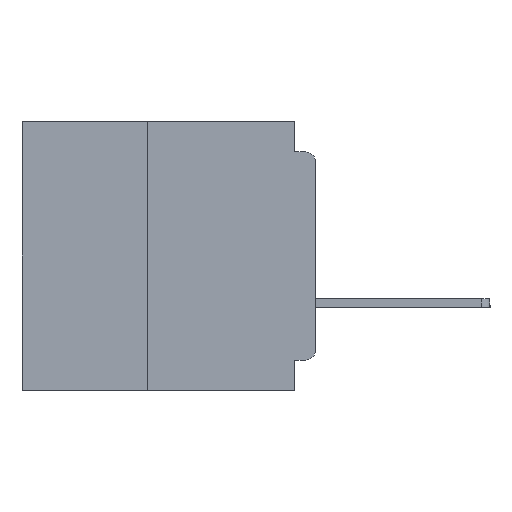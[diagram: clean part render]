
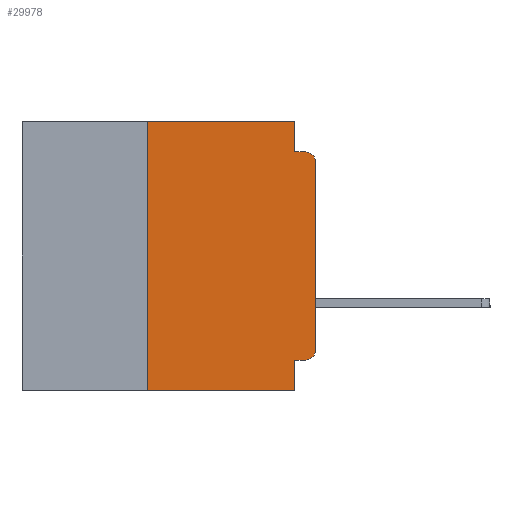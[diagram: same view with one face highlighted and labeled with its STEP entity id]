
A CAD part, left-side view. The second image highlights one B-rep face of the part: STEP entity #29978.
In plain terms, the highlighted planar face has unit normal (-1, 0, 0).
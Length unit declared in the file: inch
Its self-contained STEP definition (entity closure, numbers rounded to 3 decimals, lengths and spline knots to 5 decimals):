
#248 = VERTEX_POINT ( 'NONE', #37968 ) ;
#346 = LINE ( 'NONE', #29922, #40143 ) ;
#841 = CARTESIAN_POINT ( 'NONE',  ( 0., 0.015, -0.06 ) ) ;
#1533 = CARTESIAN_POINT ( 'NONE',  ( 0., 0.25, 0. ) ) ;
#1706 = ORIENTED_EDGE ( 'NONE', *, *, #34268, .T. ) ;
#2144 = EDGE_CURVE ( 'NONE', #54916, #248, #28563, .T. ) ;
#3180 = VECTOR ( 'NONE', #64614, 39.37008 ) ;
#4664 = ORIENTED_EDGE ( 'NONE', *, *, #55768, .F. ) ;
#5012 = CARTESIAN_POINT ( 'NONE',  ( 0., 0.015, -0.355 ) ) ;
#5513 = VECTOR ( 'NONE', #36241, 39.37008 ) ;
#5719 = VECTOR ( 'NONE', #46419, 39.37008 ) ;
#5851 = CARTESIAN_POINT ( 'NONE',  ( 0., 0.015, -0.045 ) ) ;
#6122 = DIRECTION ( 'NONE',  ( 0., 0., -1. ) ) ;
#8767 = LINE ( 'NONE', #56888, #5513 ) ;
#10810 = CARTESIAN_POINT ( 'NONE',  ( 0., 0., -0.06 ) ) ;
#13186 = VECTOR ( 'NONE', #66422, 39.37008 ) ;
#15886 = EDGE_CURVE ( 'NONE', #248, #17836, #17030, .T. ) ;
#16548 = DIRECTION ( 'NONE',  ( 1., 0., 0. ) ) ;
#17030 = LINE ( 'NONE', #44818, #20254 ) ;
#17603 = ORIENTED_EDGE ( 'NONE', *, *, #54045, .F. ) ;
#17836 = VERTEX_POINT ( 'NONE', #18059 ) ;
#18059 = CARTESIAN_POINT ( 'NONE',  ( 0., 0.031, -0.4 ) ) ;
#18312 = AXIS2_PLACEMENT_3D ( 'NONE', #22030, #58297, #27219 ) ;
#19252 = DIRECTION ( 'NONE',  ( 0., 0., -1. ) ) ;
#19547 = LINE ( 'NONE', #51428, #5719 ) ;
#20254 = VECTOR ( 'NONE', #19252, 39.37008 ) ;
#21035 = VERTEX_POINT ( 'NONE', #61242 ) ;
#22030 = CARTESIAN_POINT ( 'NONE',  ( 0., 0.015, -0.34 ) ) ;
#23277 = ORIENTED_EDGE ( 'NONE', *, *, #52004, .T. ) ;
#24165 = EDGE_CURVE ( 'NONE', #42145, #42224, #346, .T. ) ;
#26430 = VERTEX_POINT ( 'NONE', #1533 ) ;
#27219 = DIRECTION ( 'NONE',  ( 0., 0., -1. ) ) ;
#27846 = CARTESIAN_POINT ( 'NONE',  ( 0., 0.031, 0. ) ) ;
#28563 = LINE ( 'NONE', #45722, #13186 ) ;
#29922 = CARTESIAN_POINT ( 'NONE',  ( 0., 0., -0.045 ) ) ;
#29978 = ADVANCED_FACE ( 'NONE', ( #32818 ), #37120, .F. ) ;
#30312 = ORIENTED_EDGE ( 'NONE', *, *, #15886, .F. ) ;
#31312 = ORIENTED_EDGE ( 'NONE', *, *, #24165, .F. ) ;
#32818 = FACE_OUTER_BOUND ( 'NONE', #62826, .T. ) ;
#33409 = VECTOR ( 'NONE', #45079, 39.37008 ) ;
#34268 = EDGE_CURVE ( 'NONE', #21035, #17836, #8767, .T. ) ;
#34377 = VERTEX_POINT ( 'NONE', #10810 ) ;
#36174 = CIRCLE ( 'NONE', #65828, 0.015 ) ;
#36241 = DIRECTION ( 'NONE',  ( 0., -1., 0. ) ) ;
#36369 = EDGE_CURVE ( 'NONE', #21035, #26430, #41226, .T. ) ;
#37120 = PLANE ( 'NONE',  #41165 ) ;
#37164 = DIRECTION ( 'NONE',  ( -1., 0., 0. ) ) ;
#37672 = EDGE_CURVE ( 'NONE', #34377, #42224, #36174, .T. ) ;
#37968 = CARTESIAN_POINT ( 'NONE',  ( 0., 0.031, -0.355 ) ) ;
#39195 = ORIENTED_EDGE ( 'NONE', *, *, #55540, .T. ) ;
#40143 = VECTOR ( 'NONE', #55816, 39.37008 ) ;
#41165 = AXIS2_PLACEMENT_3D ( 'NONE', #47565, #16548, #52769 ) ;
#41226 = LINE ( 'NONE', #58347, #67251 ) ;
#42145 = VERTEX_POINT ( 'NONE', #46649 ) ;
#42224 = VERTEX_POINT ( 'NONE', #5851 ) ;
#44596 = LINE ( 'NONE', #58444, #3180 ) ;
#44760 = VERTEX_POINT ( 'NONE', #45017 ) ;
#44818 = CARTESIAN_POINT ( 'NONE',  ( 0., 0.031, -0.4 ) ) ;
#45017 = CARTESIAN_POINT ( 'NONE',  ( 0., 0., -0.34 ) ) ;
#45079 = DIRECTION ( 'NONE',  ( 0., -1., 0. ) ) ;
#45722 = CARTESIAN_POINT ( 'NONE',  ( 0., 0., -0.355 ) ) ;
#46419 = DIRECTION ( 'NONE',  ( 0., 0., 1. ) ) ;
#46649 = CARTESIAN_POINT ( 'NONE',  ( 0., 0.031, -0.045 ) ) ;
#47565 = CARTESIAN_POINT ( 'NONE',  ( 0., 0.437, 0. ) ) ;
#51428 = CARTESIAN_POINT ( 'NONE',  ( 0., 0., 0. ) ) ;
#52004 = EDGE_CURVE ( 'NONE', #54916, #44760, #58487, .T. ) ;
#52769 = DIRECTION ( 'NONE',  ( 0., 0., -1. ) ) ;
#54045 = EDGE_CURVE ( 'NONE', #26430, #66550, #64300, .T. ) ;
#54916 = VERTEX_POINT ( 'NONE', #5012 ) ;
#55540 = EDGE_CURVE ( 'NONE', #44760, #34377, #19547, .T. ) ;
#55768 = EDGE_CURVE ( 'NONE', #66550, #42145, #44596, .T. ) ;
#55816 = DIRECTION ( 'NONE',  ( 0., -1., 0. ) ) ;
#56888 = CARTESIAN_POINT ( 'NONE',  ( 0., 0.437, -0.4 ) ) ;
#58297 = DIRECTION ( 'NONE',  ( -1., 0., 0. ) ) ;
#58347 = CARTESIAN_POINT ( 'NONE',  ( 0., 0.25, -0.4 ) ) ;
#58444 = CARTESIAN_POINT ( 'NONE',  ( 0., 0.031, 0. ) ) ;
#58487 = CIRCLE ( 'NONE', #18312, 0.015 ) ;
#58708 = ORIENTED_EDGE ( 'NONE', *, *, #2144, .F. ) ;
#61242 = CARTESIAN_POINT ( 'NONE',  ( 0., 0.25, -0.4 ) ) ;
#62826 = EDGE_LOOP ( 'NONE', ( #39195, #64158, #31312, #4664, #17603, #64123, #1706, #30312, #58708, #23277 ) ) ;
#63603 = DIRECTION ( 'NONE',  ( 0., 0., 1. ) ) ;
#64123 = ORIENTED_EDGE ( 'NONE', *, *, #36369, .F. ) ;
#64158 = ORIENTED_EDGE ( 'NONE', *, *, #37672, .T. ) ;
#64300 = LINE ( 'NONE', #65783, #33409 ) ;
#64614 = DIRECTION ( 'NONE',  ( 0., 0., -1. ) ) ;
#65783 = CARTESIAN_POINT ( 'NONE',  ( 0., 0.437, 0. ) ) ;
#65828 = AXIS2_PLACEMENT_3D ( 'NONE', #841, #37164, #6122 ) ;
#66422 = DIRECTION ( 'NONE',  ( 0., 1., 0. ) ) ;
#66550 = VERTEX_POINT ( 'NONE', #27846 ) ;
#67251 = VECTOR ( 'NONE', #63603, 39.37008 ) ;
